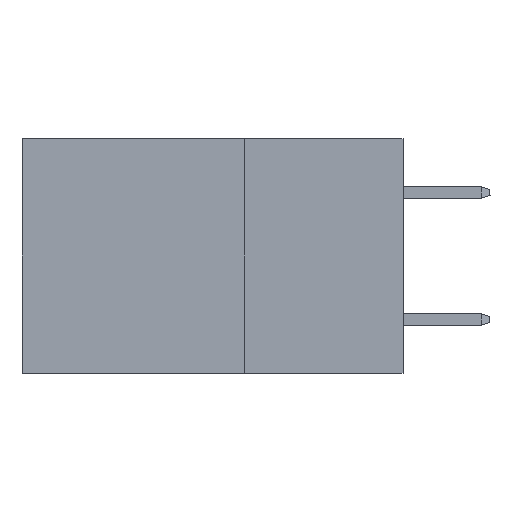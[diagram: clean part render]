
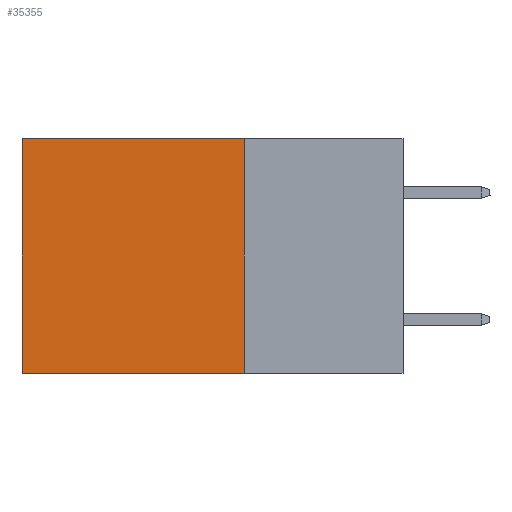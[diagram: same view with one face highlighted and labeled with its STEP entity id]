
A CAD part, left-side view. The second image highlights one B-rep face of the part: STEP entity #35355.
In plain terms, the highlighted planar face has unit normal (-1, 0, 0).
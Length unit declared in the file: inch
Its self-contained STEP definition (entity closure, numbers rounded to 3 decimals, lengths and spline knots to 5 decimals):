
#1387 = EDGE_LOOP ( 'NONE', ( #41137, #42376, #31787, #27211 ) ) ;
#1974 = CARTESIAN_POINT ( 'NONE',  ( 0.2875, 0.6, 0. ) ) ;
#3177 = DIRECTION ( 'NONE',  ( 0., 1., 0. ) ) ;
#5771 = FACE_OUTER_BOUND ( 'NONE', #1387, .T. ) ;
#6960 = EDGE_CURVE ( 'NONE', #16703, #23695, #26866, .T. ) ;
#7085 = DIRECTION ( 'NONE',  ( 0., 0., -1. ) ) ;
#9953 = AXIS2_PLACEMENT_3D ( 'NONE', #36042, #22438, #38898 ) ;
#11404 = LINE ( 'NONE', #1974, #36357 ) ;
#11566 = EDGE_CURVE ( 'NONE', #35384, #16703, #19594, .T. ) ;
#15316 = DIRECTION ( 'NONE',  ( 0., 0., -1. ) ) ;
#16703 = VERTEX_POINT ( 'NONE', #26302 ) ;
#16963 = CARTESIAN_POINT ( 'NONE',  ( 0.2875, 0.25, -0.37 ) ) ;
#19355 = CARTESIAN_POINT ( 'NONE',  ( 0.2875, 0.25, 0. ) ) ;
#19594 = LINE ( 'NONE', #32999, #30499 ) ;
#21498 = LINE ( 'NONE', #41265, #27597 ) ;
#22002 = CARTESIAN_POINT ( 'NONE',  ( 0.2875, 0.6, 0. ) ) ;
#22438 = DIRECTION ( 'NONE',  ( 1., 0., 0. ) ) ;
#23695 = VERTEX_POINT ( 'NONE', #37947 ) ;
#25535 = VERTEX_POINT ( 'NONE', #22002 ) ;
#26302 = CARTESIAN_POINT ( 'NONE',  ( 0.2875, 0.25, -0.37 ) ) ;
#26866 = LINE ( 'NONE', #16963, #35922 ) ;
#27211 = ORIENTED_EDGE ( 'NONE', *, *, #36895, .T. ) ;
#27597 = VECTOR ( 'NONE', #27678, 39.37008 ) ;
#27678 = DIRECTION ( 'NONE',  ( 0., 1., 0. ) ) ;
#30499 = VECTOR ( 'NONE', #7085, 39.37008 ) ;
#31787 = ORIENTED_EDGE ( 'NONE', *, *, #11566, .F. ) ;
#32999 = CARTESIAN_POINT ( 'NONE',  ( 0.2875, 0.25, 0. ) ) ;
#35355 = ADVANCED_FACE ( 'NONE', ( #5771 ), #35605, .F. ) ;
#35384 = VERTEX_POINT ( 'NONE', #19355 ) ;
#35605 = PLANE ( 'NONE',  #9953 ) ;
#35922 = VECTOR ( 'NONE', #3177, 39.37008 ) ;
#36042 = CARTESIAN_POINT ( 'NONE',  ( 0.2875, 0.25, 0. ) ) ;
#36357 = VECTOR ( 'NONE', #15316, 39.37008 ) ;
#36895 = EDGE_CURVE ( 'NONE', #35384, #25535, #21498, .T. ) ;
#37947 = CARTESIAN_POINT ( 'NONE',  ( 0.2875, 0.6, -0.37 ) ) ;
#38898 = DIRECTION ( 'NONE',  ( 0., 0., -1. ) ) ;
#41137 = ORIENTED_EDGE ( 'NONE', *, *, #42000, .T. ) ;
#41265 = CARTESIAN_POINT ( 'NONE',  ( 0.2875, 0.25, 0. ) ) ;
#42000 = EDGE_CURVE ( 'NONE', #25535, #23695, #11404, .T. ) ;
#42376 = ORIENTED_EDGE ( 'NONE', *, *, #6960, .F. ) ;
